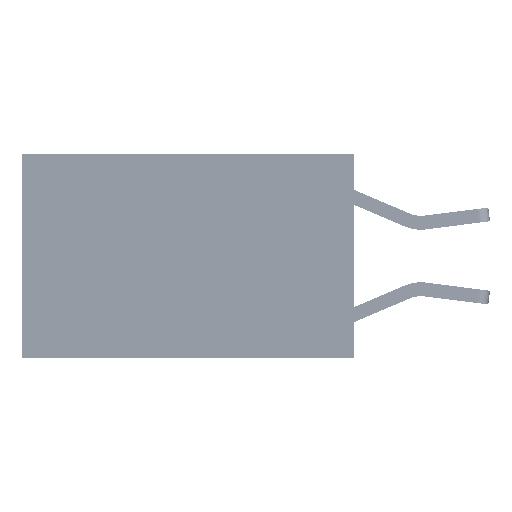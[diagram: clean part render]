
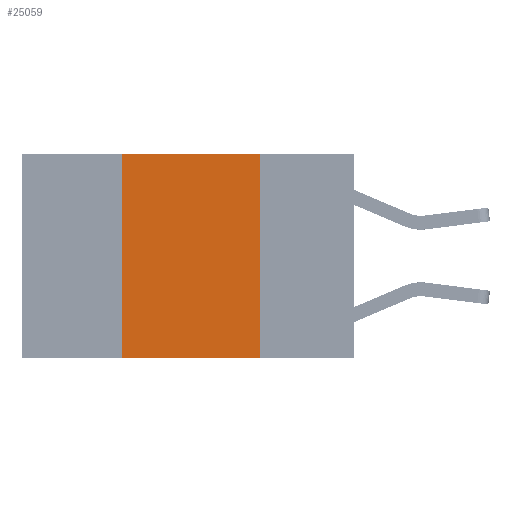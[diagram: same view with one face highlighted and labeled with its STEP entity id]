
A CAD part, left-side view. The second image highlights one B-rep face of the part: STEP entity #25059.
In plain terms, the highlighted planar face has unit normal (-1, 0, 0).
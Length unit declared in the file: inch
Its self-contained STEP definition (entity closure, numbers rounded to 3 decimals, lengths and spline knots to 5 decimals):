
#474 = VERTEX_POINT ( 'NONE', #7955 ) ;
#2336 = ORIENTED_EDGE ( 'NONE', *, *, #8008, .F. ) ;
#3143 = ORIENTED_EDGE ( 'NONE', *, *, #27935, .F. ) ;
#3347 = CARTESIAN_POINT ( 'NONE',  ( 0., 0.42, 0. ) ) ;
#4690 = VERTEX_POINT ( 'NONE', #32253 ) ;
#4863 = VECTOR ( 'NONE', #5897, 39.37008 ) ;
#5739 = CARTESIAN_POINT ( 'NONE',  ( 0., 0.6, -0.37 ) ) ;
#5897 = DIRECTION ( 'NONE',  ( 0., 0., 1. ) ) ;
#6721 = LINE ( 'NONE', #28688, #19404 ) ;
#7319 = CARTESIAN_POINT ( 'NONE',  ( 0., 0.17, 0. ) ) ;
#7955 = CARTESIAN_POINT ( 'NONE',  ( 0., 0.42, -0.37 ) ) ;
#8008 = EDGE_CURVE ( 'NONE', #13347, #4690, #24889, .T. ) ;
#8309 = EDGE_CURVE ( 'NONE', #474, #4690, #23679, .T. ) ;
#9108 = ORIENTED_EDGE ( 'NONE', *, *, #29929, .F. ) ;
#9114 = FACE_OUTER_BOUND ( 'NONE', #9184, .T. ) ;
#9184 = EDGE_LOOP ( 'NONE', ( #2336, #9108, #3143, #17430 ) ) ;
#11696 = VERTEX_POINT ( 'NONE', #13763 ) ;
#11946 = CARTESIAN_POINT ( 'NONE',  ( 0., 0.6, 0. ) ) ;
#13347 = VERTEX_POINT ( 'NONE', #18963 ) ;
#13763 = CARTESIAN_POINT ( 'NONE',  ( 0., 0.42, 0. ) ) ;
#16972 = VECTOR ( 'NONE', #18361, 39.37008 ) ;
#17061 = DIRECTION ( 'NONE',  ( 0., 0., -1. ) ) ;
#17430 = ORIENTED_EDGE ( 'NONE', *, *, #8309, .T. ) ;
#18166 = VECTOR ( 'NONE', #20051, 39.37008 ) ;
#18361 = DIRECTION ( 'NONE',  ( 0., -1., 0. ) ) ;
#18963 = CARTESIAN_POINT ( 'NONE',  ( 0., 0.17, 0. ) ) ;
#19404 = VECTOR ( 'NONE', #31202, 39.37008 ) ;
#20051 = DIRECTION ( 'NONE',  ( 0., 0., -1. ) ) ;
#23679 = LINE ( 'NONE', #5739, #16972 ) ;
#24889 = LINE ( 'NONE', #7319, #18166 ) ;
#25054 = LINE ( 'NONE', #3347, #4863 ) ;
#25059 = ADVANCED_FACE ( 'NONE', ( #9114 ), #29627, .F. ) ;
#27935 = EDGE_CURVE ( 'NONE', #474, #11696, #25054, .T. ) ;
#28688 = CARTESIAN_POINT ( 'NONE',  ( 0., 0.6, 0. ) ) ;
#29627 = PLANE ( 'NONE',  #31611 ) ;
#29929 = EDGE_CURVE ( 'NONE', #11696, #13347, #6721, .T. ) ;
#31202 = DIRECTION ( 'NONE',  ( 0., -1., 0. ) ) ;
#31611 = AXIS2_PLACEMENT_3D ( 'NONE', #11946, #32150, #17061 ) ;
#32150 = DIRECTION ( 'NONE',  ( 1., 0., 0. ) ) ;
#32253 = CARTESIAN_POINT ( 'NONE',  ( 0., 0.17, -0.37 ) ) ;
